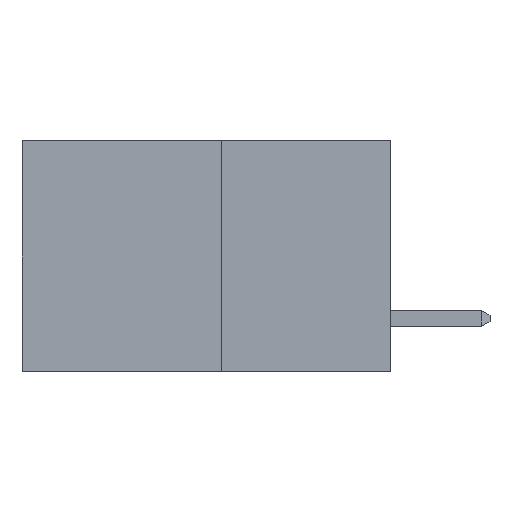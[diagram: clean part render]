
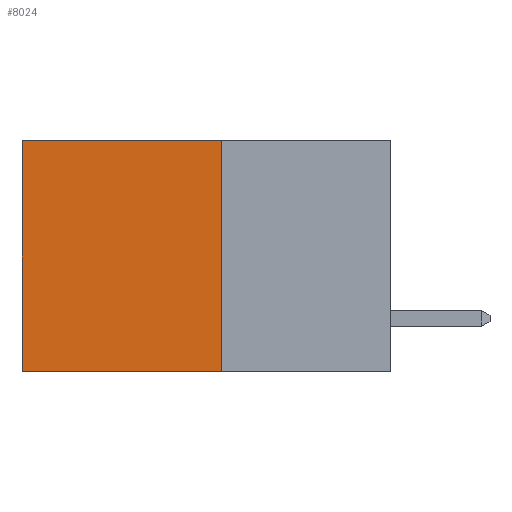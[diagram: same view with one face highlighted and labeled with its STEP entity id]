
A CAD part, left-side view. The second image highlights one B-rep face of the part: STEP entity #8024.
In plain terms, the highlighted planar face has unit normal (-1, 0, 0).
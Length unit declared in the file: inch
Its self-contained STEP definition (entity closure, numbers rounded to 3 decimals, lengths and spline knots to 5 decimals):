
#94 = DIRECTION ( 'NONE',  ( 0., 0., -1. ) ) ;
#318 = CARTESIAN_POINT ( 'NONE',  ( 0.277, 0.59, -0.37 ) ) ;
#492 = EDGE_CURVE ( 'NONE', #6375, #4091, #7579, .T. ) ;
#925 = VECTOR ( 'NONE', #2669, 39.37008 ) ;
#1005 = DIRECTION ( 'NONE',  ( 0., 0., -1. ) ) ;
#1310 = EDGE_CURVE ( 'NONE', #10033, #4091, #10485, .T. ) ;
#1314 = CARTESIAN_POINT ( 'NONE',  ( 0.277, 0.59, -0.37 ) ) ;
#1415 = LINE ( 'NONE', #1853, #9950 ) ;
#1853 = CARTESIAN_POINT ( 'NONE',  ( 0.277, 0.27, 0. ) ) ;
#2116 = DIRECTION ( 'NONE',  ( 0., 0., -1. ) ) ;
#2591 = CARTESIAN_POINT ( 'NONE',  ( 0.277, 0.27, -0.37 ) ) ;
#2634 = CARTESIAN_POINT ( 'NONE',  ( 0.277, 0.27, -0.37 ) ) ;
#2669 = DIRECTION ( 'NONE',  ( 0., 1., 0. ) ) ;
#3434 = ORIENTED_EDGE ( 'NONE', *, *, #8701, .T. ) ;
#3743 = CARTESIAN_POINT ( 'NONE',  ( 0.277, 0.27, -0.37 ) ) ;
#4001 = FACE_OUTER_BOUND ( 'NONE', #8160, .T. ) ;
#4091 = VERTEX_POINT ( 'NONE', #318 ) ;
#4587 = CARTESIAN_POINT ( 'NONE',  ( 0.277, 0.27, 0. ) ) ;
#5132 = DIRECTION ( 'NONE',  ( 1., 0., 0. ) ) ;
#5407 = CARTESIAN_POINT ( 'NONE',  ( 0.277, 0.59, 0. ) ) ;
#6375 = VERTEX_POINT ( 'NONE', #8895 ) ;
#6995 = VERTEX_POINT ( 'NONE', #4587 ) ;
#7579 = LINE ( 'NONE', #2591, #925 ) ;
#7998 = VECTOR ( 'NONE', #2116, 39.37008 ) ;
#8024 = ADVANCED_FACE ( 'NONE', ( #4001 ), #10076, .F. ) ;
#8160 = EDGE_LOOP ( 'NONE', ( #8557, #8825, #8716, #3434 ) ) ;
#8331 = VECTOR ( 'NONE', #1005, 39.37008 ) ;
#8557 = ORIENTED_EDGE ( 'NONE', *, *, #1310, .T. ) ;
#8701 = EDGE_CURVE ( 'NONE', #6995, #10033, #1415, .T. ) ;
#8716 = ORIENTED_EDGE ( 'NONE', *, *, #8899, .F. ) ;
#8825 = ORIENTED_EDGE ( 'NONE', *, *, #492, .F. ) ;
#8895 = CARTESIAN_POINT ( 'NONE',  ( 0.277, 0.27, -0.37 ) ) ;
#8899 = EDGE_CURVE ( 'NONE', #6995, #6375, #10151, .T. ) ;
#9126 = AXIS2_PLACEMENT_3D ( 'NONE', #2634, #5132, #94 ) ;
#9313 = DIRECTION ( 'NONE',  ( 0., 1., 0. ) ) ;
#9950 = VECTOR ( 'NONE', #9313, 39.37008 ) ;
#10033 = VERTEX_POINT ( 'NONE', #5407 ) ;
#10076 = PLANE ( 'NONE',  #9126 ) ;
#10151 = LINE ( 'NONE', #3743, #7998 ) ;
#10485 = LINE ( 'NONE', #1314, #8331 ) ;
